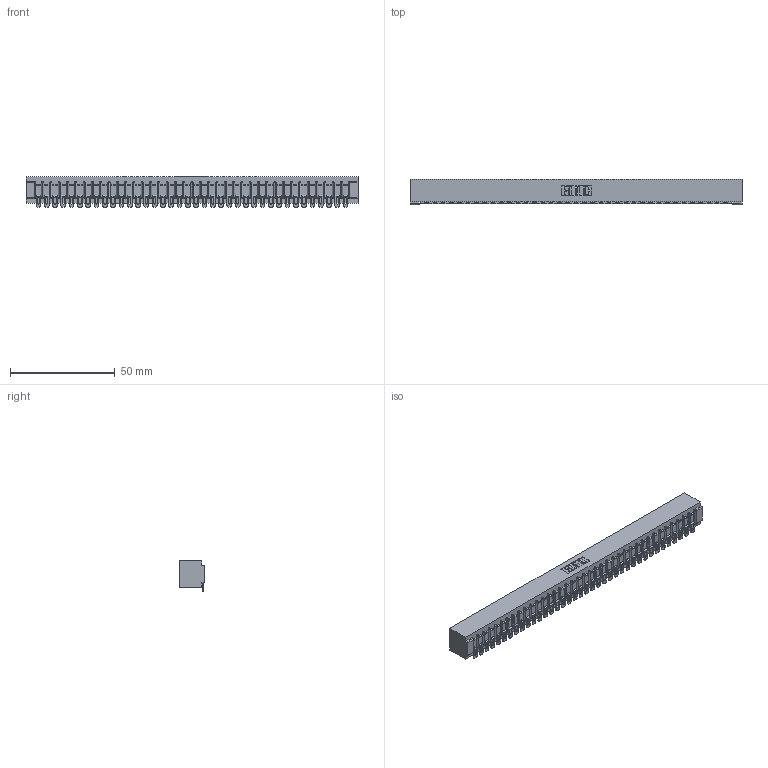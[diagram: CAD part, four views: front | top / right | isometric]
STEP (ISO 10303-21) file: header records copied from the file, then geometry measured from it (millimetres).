
FILE_DESCRIPTION (( 'STEP AP203' ), '1' );
FILE_NAME ('307-038-454-101.STEP', '2020-09-29T06:33:38', ( '' ), ( '' ), 'SwSTEP 2.0', 'SolidWorks 2020', '' );
FILE_SCHEMA (( 'CONFIG_CONTROL_DESIGN' ));
Length unit declared in the file: inch
Products named in the file (3): 307-290-002_554; 307 Part_No Mounting Lugs; 307-038-454-101
Assembly tree (39 placements, depth 2):
  307-038-454-101
    307 Part_No Mounting Lugs
    307-290-002_554  x38
Bounding box: 158.45 x 12.01 x 14.52 mm (x, y, z)
Volume: 17497.3 mm3; surface area: 22408.7 mm2
Topology: 39 solids, 39 shells, 3227 faces, 9913 edges, 6502 vertices
Faces by surface type: plane 1814, cylinder 1335, sphere 78
Entity records: 33757 total; most frequent: CARTESIAN_POINT 5694, ORIENTED_EDGE 5684, DIRECTION 5538, EDGE_CURVE 2842, LINE 2170, VECTOR 2170, VERTEX_POINT 1840, AXIS2_PLACEMENT_3D 1684
